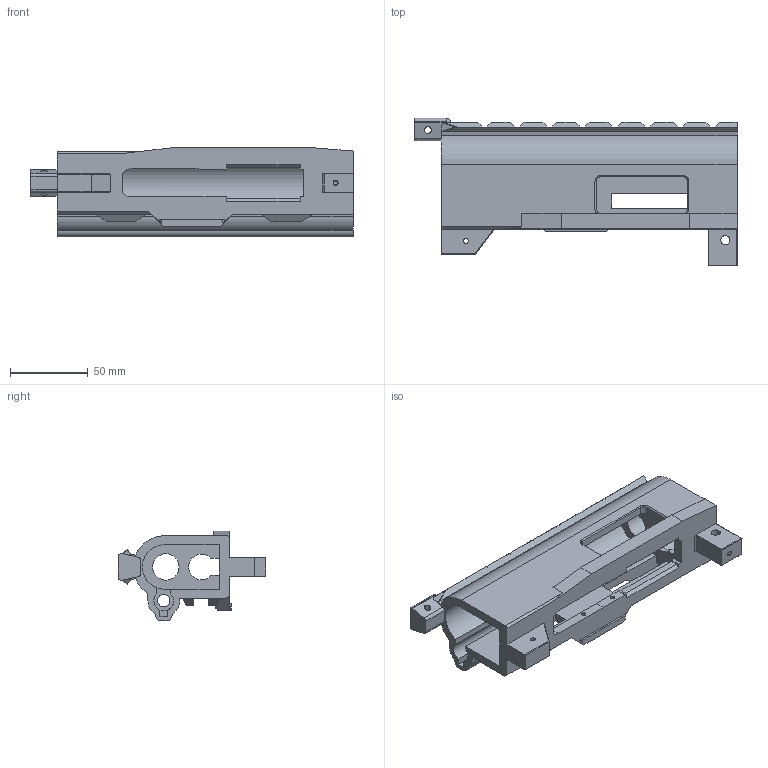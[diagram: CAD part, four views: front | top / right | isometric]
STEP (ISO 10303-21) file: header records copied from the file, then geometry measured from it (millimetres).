
FILE_DESCRIPTION(('STEP AP214'),'1');
FILE_NAME('MOD9E Upper Receiver.stp','2020-09-01T22:16:56',(' '),(' '),'Spatial InterOp 3D',' ',' ');
FILE_SCHEMA(('AUTOMOTIVE_DESIGN { 1 0 10303 214 1 1 1 1 }'));
Length unit declared in the file: metre
Products named in the file (1): Solid
Bounding box: 207.36 x 94.9 x 57.79 mm (x, y, z)
Volume: 240504.1 mm3; surface area: 84764.4 mm2
Topology: 1 solids, 1 shells, 257 faces, 698 edges, 448 vertices
Faces by surface type: plane 179, cylinder 58, cone 16, bspline 4
Entity records: 8301 total; most frequent: CARTESIAN_POINT 1699, ORIENTED_EDGE 1396, DIRECTION 1319, EDGE_CURVE 698, LINE 541, VECTOR 541, VERTEX_POINT 448, AXIS2_PLACEMENT_3D 389
